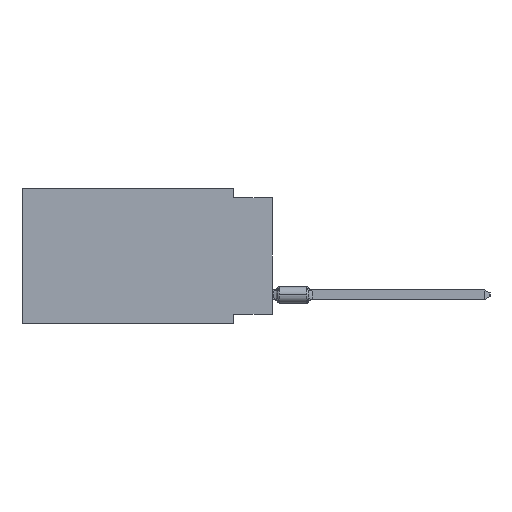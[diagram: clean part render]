
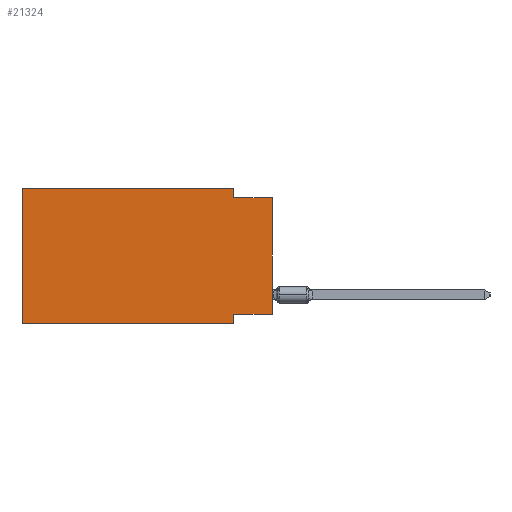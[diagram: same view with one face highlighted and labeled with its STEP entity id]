
A CAD part, left-side view. The second image highlights one B-rep face of the part: STEP entity #21324.
In plain terms, the highlighted planar face has unit normal (-1, 0, 0).
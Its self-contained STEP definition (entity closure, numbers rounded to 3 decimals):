
#2045 = DIRECTION ( 'NONE',  ( 0., 0., 1. ) ) ;
#2693 = VERTEX_POINT ( 'NONE', #14273 ) ;
#3574 = CARTESIAN_POINT ( 'NONE',  ( 0., 0., -8.255 ) ) ;
#4304 = VECTOR ( 'NONE', #2045, 1000. ) ;
#4810 = VECTOR ( 'NONE', #26051, 1000. ) ;
#5675 = CARTESIAN_POINT ( 'NONE',  ( 0., 16.383, 0. ) ) ;
#6145 = PLANE ( 'NONE',  #28316 ) ;
#6829 = LINE ( 'NONE', #13913, #29999 ) ;
#7118 = CARTESIAN_POINT ( 'NONE',  ( 0., 2.54, -8.89 ) ) ;
#7884 = EDGE_CURVE ( 'NONE', #2693, #20884, #11664, .T. ) ;
#9160 = EDGE_CURVE ( 'NONE', #28737, #20143, #23569, .T. ) ;
#9309 = LINE ( 'NONE', #19036, #17086 ) ;
#9695 = LINE ( 'NONE', #14465, #4810 ) ;
#10511 = ORIENTED_EDGE ( 'NONE', *, *, #22671, .F. ) ;
#11173 = VECTOR ( 'NONE', #18222, 1000. ) ;
#11664 = LINE ( 'NONE', #18595, #11838 ) ;
#11838 = VECTOR ( 'NONE', #30477, 1000. ) ;
#12890 = CARTESIAN_POINT ( 'NONE',  ( 0., 0., -8.255 ) ) ;
#13405 = CARTESIAN_POINT ( 'NONE',  ( 0., 16.383, 0. ) ) ;
#13544 = VERTEX_POINT ( 'NONE', #28102 ) ;
#13913 = CARTESIAN_POINT ( 'NONE',  ( 0., 0., -0.635 ) ) ;
#14273 = CARTESIAN_POINT ( 'NONE',  ( 0., 16.383, -8.89 ) ) ;
#14465 = CARTESIAN_POINT ( 'NONE',  ( 0., 2.54, 0. ) ) ;
#16381 = DIRECTION ( 'NONE',  ( 0., -1., 0. ) ) ;
#17032 = ORIENTED_EDGE ( 'NONE', *, *, #7884, .F. ) ;
#17086 = VECTOR ( 'NONE', #21507, 1000. ) ;
#17568 = VERTEX_POINT ( 'NONE', #24759 ) ;
#17711 = EDGE_CURVE ( 'NONE', #20143, #22039, #9309, .T. ) ;
#18163 = DIRECTION ( 'NONE',  ( 0., -1., 0. ) ) ;
#18204 = EDGE_CURVE ( 'NONE', #28737, #17568, #20120, .T. ) ;
#18222 = DIRECTION ( 'NONE',  ( 0., -1., 0. ) ) ;
#18595 = CARTESIAN_POINT ( 'NONE',  ( 0., 16.383, 0. ) ) ;
#19036 = CARTESIAN_POINT ( 'NONE',  ( 0., 2.54, -8.89 ) ) ;
#20120 = LINE ( 'NONE', #24752, #4304 ) ;
#20143 = VERTEX_POINT ( 'NONE', #29114 ) ;
#20564 = ORIENTED_EDGE ( 'NONE', *, *, #17711, .F. ) ;
#20884 = VERTEX_POINT ( 'NONE', #13405 ) ;
#21004 = LINE ( 'NONE', #22855, #11173 ) ;
#21324 = ADVANCED_FACE ( 'NONE', ( #27257 ), #6145, .F. ) ;
#21507 = DIRECTION ( 'NONE',  ( 0., 0., -1. ) ) ;
#22002 = VERTEX_POINT ( 'NONE', #22397 ) ;
#22039 = VERTEX_POINT ( 'NONE', #7118 ) ;
#22069 = EDGE_CURVE ( 'NONE', #2693, #22039, #21004, .T. ) ;
#22397 = CARTESIAN_POINT ( 'NONE',  ( 0., 2.54, 0. ) ) ;
#22671 = EDGE_CURVE ( 'NONE', #22002, #13544, #9695, .T. ) ;
#22791 = DIRECTION ( 'NONE',  ( 1., 0., 0. ) ) ;
#22855 = CARTESIAN_POINT ( 'NONE',  ( 0., 16.383, -8.89 ) ) ;
#23569 = LINE ( 'NONE', #12890, #28138 ) ;
#23957 = ORIENTED_EDGE ( 'NONE', *, *, #22069, .T. ) ;
#24315 = DIRECTION ( 'NONE',  ( 0., 1., 0. ) ) ;
#24752 = CARTESIAN_POINT ( 'NONE',  ( 0., 0., 0. ) ) ;
#24759 = CARTESIAN_POINT ( 'NONE',  ( 0., 0., -0.635 ) ) ;
#25143 = VECTOR ( 'NONE', #18163, 1000. ) ;
#25251 = LINE ( 'NONE', #29885, #25143 ) ;
#25993 = EDGE_LOOP ( 'NONE', ( #28644, #26022, #10511, #27143, #17032, #23957, #20564, #27720 ) ) ;
#26022 = ORIENTED_EDGE ( 'NONE', *, *, #28519, .F. ) ;
#26051 = DIRECTION ( 'NONE',  ( 0., 0., -1. ) ) ;
#26297 = EDGE_CURVE ( 'NONE', #20884, #22002, #25251, .T. ) ;
#27107 = DIRECTION ( 'NONE',  ( 0., 0., -1. ) ) ;
#27143 = ORIENTED_EDGE ( 'NONE', *, *, #26297, .F. ) ;
#27257 = FACE_OUTER_BOUND ( 'NONE', #25993, .T. ) ;
#27720 = ORIENTED_EDGE ( 'NONE', *, *, #9160, .F. ) ;
#28102 = CARTESIAN_POINT ( 'NONE',  ( 0., 2.54, -0.635 ) ) ;
#28138 = VECTOR ( 'NONE', #24315, 1000. ) ;
#28316 = AXIS2_PLACEMENT_3D ( 'NONE', #5675, #22791, #27107 ) ;
#28519 = EDGE_CURVE ( 'NONE', #13544, #17568, #6829, .T. ) ;
#28644 = ORIENTED_EDGE ( 'NONE', *, *, #18204, .T. ) ;
#28737 = VERTEX_POINT ( 'NONE', #3574 ) ;
#29114 = CARTESIAN_POINT ( 'NONE',  ( 0., 2.54, -8.255 ) ) ;
#29885 = CARTESIAN_POINT ( 'NONE',  ( 0., 16.383, 0. ) ) ;
#29999 = VECTOR ( 'NONE', #16381, 1000. ) ;
#30477 = DIRECTION ( 'NONE',  ( 0., 0., 1. ) ) ;
